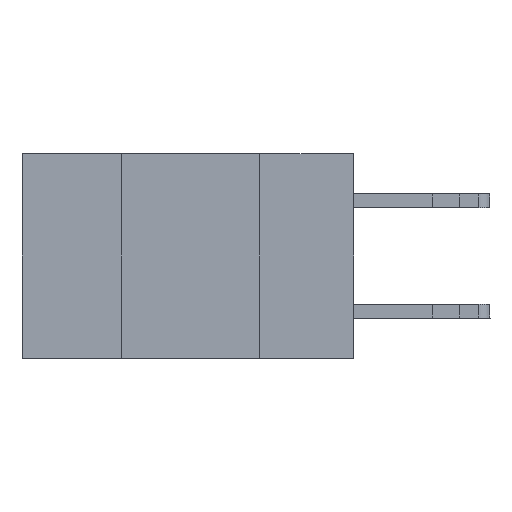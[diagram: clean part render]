
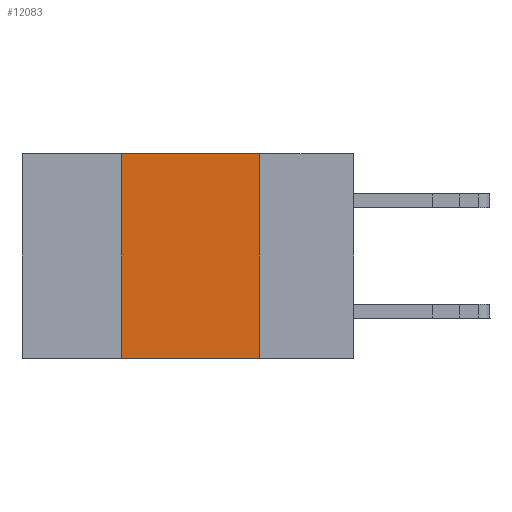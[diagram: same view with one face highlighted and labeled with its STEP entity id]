
A CAD part, left-side view. The second image highlights one B-rep face of the part: STEP entity #12083.
In plain terms, the highlighted planar face has unit normal (-1, 0, 0).
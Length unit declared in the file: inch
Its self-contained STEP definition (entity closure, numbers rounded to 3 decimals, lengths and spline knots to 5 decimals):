
#402 = ORIENTED_EDGE ( 'NONE', *, *, #21391, .F. ) ;
#592 = CARTESIAN_POINT ( 'NONE',  ( 0., 0.42, 0. ) ) ;
#845 = CARTESIAN_POINT ( 'NONE',  ( 0., 0.6, 0. ) ) ;
#1040 = VECTOR ( 'NONE', #14331, 39.37008 ) ;
#1988 = ORIENTED_EDGE ( 'NONE', *, *, #14820, .F. ) ;
#2060 = ORIENTED_EDGE ( 'NONE', *, *, #16552, .T. ) ;
#2263 = LINE ( 'NONE', #12495, #1040 ) ;
#2809 = DIRECTION ( 'NONE',  ( 0., 0., -1. ) ) ;
#3077 = CARTESIAN_POINT ( 'NONE',  ( 0., 0.42, -0.37 ) ) ;
#3326 = EDGE_CURVE ( 'NONE', #7644, #4319, #2263, .T. ) ;
#3484 = ORIENTED_EDGE ( 'NONE', *, *, #3326, .F. ) ;
#3728 = CARTESIAN_POINT ( 'NONE',  ( 0., 0.17, -0.37 ) ) ;
#4319 = VERTEX_POINT ( 'NONE', #3728 ) ;
#5544 = CARTESIAN_POINT ( 'NONE',  ( 0., 0.6, -0.37 ) ) ;
#7644 = VERTEX_POINT ( 'NONE', #11307 ) ;
#10491 = EDGE_LOOP ( 'NONE', ( #3484, #1988, #402, #2060 ) ) ;
#10578 = PLANE ( 'NONE',  #20060 ) ;
#11307 = CARTESIAN_POINT ( 'NONE',  ( 0., 0.17, 0. ) ) ;
#12083 = ADVANCED_FACE ( 'NONE', ( #14137 ), #10578, .F. ) ;
#12495 = CARTESIAN_POINT ( 'NONE',  ( 0., 0.17, 0. ) ) ;
#13369 = VECTOR ( 'NONE', #16849, 39.37008 ) ;
#13448 = VERTEX_POINT ( 'NONE', #3077 ) ;
#14137 = FACE_OUTER_BOUND ( 'NONE', #10491, .T. ) ;
#14300 = DIRECTION ( 'NONE',  ( 1., 0., 0. ) ) ;
#14331 = DIRECTION ( 'NONE',  ( 0., 0., -1. ) ) ;
#14820 = EDGE_CURVE ( 'NONE', #23638, #7644, #19122, .T. ) ;
#15021 = VECTOR ( 'NONE', #21572, 39.37008 ) ;
#16552 = EDGE_CURVE ( 'NONE', #13448, #4319, #22996, .T. ) ;
#16849 = DIRECTION ( 'NONE',  ( 0., -1., 0. ) ) ;
#18570 = VECTOR ( 'NONE', #23874, 39.37008 ) ;
#19122 = LINE ( 'NONE', #22043, #18570 ) ;
#19868 = LINE ( 'NONE', #23393, #15021 ) ;
#20060 = AXIS2_PLACEMENT_3D ( 'NONE', #845, #14300, #2809 ) ;
#21391 = EDGE_CURVE ( 'NONE', #13448, #23638, #19868, .T. ) ;
#21572 = DIRECTION ( 'NONE',  ( 0., 0., 1. ) ) ;
#22043 = CARTESIAN_POINT ( 'NONE',  ( 0., 0.6, 0. ) ) ;
#22996 = LINE ( 'NONE', #5544, #13369 ) ;
#23393 = CARTESIAN_POINT ( 'NONE',  ( 0., 0.42, 0. ) ) ;
#23638 = VERTEX_POINT ( 'NONE', #592 ) ;
#23874 = DIRECTION ( 'NONE',  ( 0., -1., 0. ) ) ;
